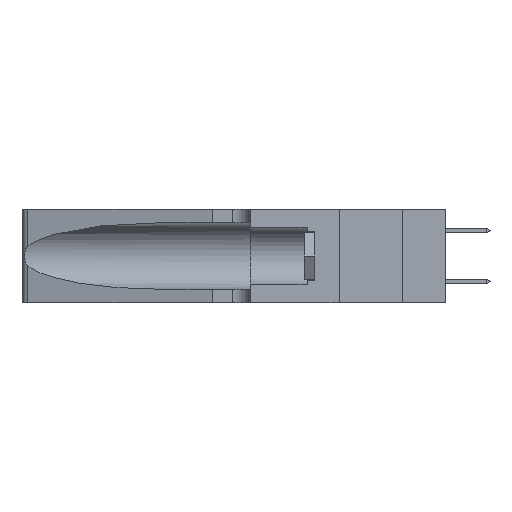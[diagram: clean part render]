
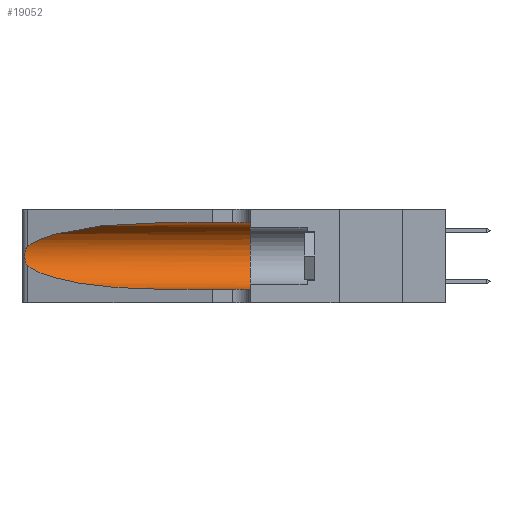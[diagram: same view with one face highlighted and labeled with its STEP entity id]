
A CAD part, left-side view. The second image highlights one B-rep face of the part: STEP entity #19052.
In plain terms, the highlighted cylindrical face has radius 3.308 mm (diameter 6.617 mm), a partial arc.
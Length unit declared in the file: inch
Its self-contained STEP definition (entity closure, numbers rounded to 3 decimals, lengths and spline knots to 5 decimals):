
#151 =( BOUNDED_CURVE ( )  B_SPLINE_CURVE ( 3, ( #10695, #19587, #8833, #23328 ),
 .UNSPECIFIED., .F., .T. ) 
 B_SPLINE_CURVE_WITH_KNOTS ( ( 4, 4 ),
 ( 1.5708, 2.84003 ),
 .UNSPECIFIED. ) 
 CURVE ( )  GEOMETRIC_REPRESENTATION_ITEM ( )  RATIONAL_B_SPLINE_CURVE ( ( 1., 0.87, 0.87, 1. ) ) 
 REPRESENTATION_ITEM ( '' )  );
#840 = CIRCLE ( 'NONE', #18734, 0.13025 ) ;
#911 =( BOUNDED_CURVE ( )  B_SPLINE_CURVE ( 3, ( #17438, #15646, #2801, #6527 ),
 .UNSPECIFIED., .F., .F. ) 
 B_SPLINE_CURVE_WITH_KNOTS ( ( 4, 4 ),
 ( 3.44316, 4.71239 ),
 .UNSPECIFIED. ) 
 CURVE ( )  GEOMETRIC_REPRESENTATION_ITEM ( )  RATIONAL_B_SPLINE_CURVE ( ( 1., 0.87, 0.87, 1. ) ) 
 REPRESENTATION_ITEM ( '' )  );
#1619 = LINE ( 'NONE', #19069, #5985 ) ;
#1751 = CARTESIAN_POINT ( 'NONE',  ( 0.1305, 0.35, 0.05475 ) ) ;
#1871 = CARTESIAN_POINT ( 'NONE',  ( 0.25639, 1.23186, 0.15144 ) ) ;
#2801 = CARTESIAN_POINT ( 'NONE',  ( 0.18966, 0.96281, 0.05475 ) ) ;
#3172 = VECTOR ( 'NONE', #9650, 39.37008 ) ;
#3465 = CYLINDRICAL_SURFACE ( 'NONE', #13192, 0.13025 ) ;
#3739 = CARTESIAN_POINT ( 'NONE',  ( 0.25487, 1.22718, 0.14631 ) ) ;
#3909 = CARTESIAN_POINT ( 'NONE',  ( 0.25856, 1.23593, 0.16098 ) ) ;
#3987 = ORIENTED_EDGE ( 'NONE', *, *, #12861, .F. ) ;
#4538 = CARTESIAN_POINT ( 'NONE',  ( 0.1305, 0.35, 0.185 ) ) ;
#5388 = ORIENTED_EDGE ( 'NONE', *, *, #22211, .T. ) ;
#5521 = CARTESIAN_POINT ( 'NONE',  ( 0.25639, 1.23184, 0.21858 ) ) ;
#5745 = EDGE_CURVE ( 'NONE', #7766, #9143, #911, .T. ) ;
#5985 = VECTOR ( 'NONE', #10089, 39.37008 ) ;
#6238 = CARTESIAN_POINT ( 'NONE',  ( 0.25487, 1.22718, 0.14631 ) ) ;
#6394 = DIRECTION ( 'NONE',  ( 0., 0., 1. ) ) ;
#6527 = CARTESIAN_POINT ( 'NONE',  ( 0.1305, 0.72297, 0.05475 ) ) ;
#6987 = DIRECTION ( 'NONE',  ( 0., -1., 0. ) ) ;
#7397 = CARTESIAN_POINT ( 'NONE',  ( 0.25854, 1.2359, 0.20912 ) ) ;
#7766 = VERTEX_POINT ( 'NONE', #6238 ) ;
#8833 = CARTESIAN_POINT ( 'NONE',  ( 0.2373, 1.15595, 0.28018 ) ) ;
#8874 = CARTESIAN_POINT ( 'NONE',  ( 0.25487, 1.22718, 0.22369 ) ) ;
#9143 = VERTEX_POINT ( 'NONE', #17431 ) ;
#9253 = CARTESIAN_POINT ( 'NONE',  ( 0.26075, 1.23896, 0.19203 ) ) ;
#9650 = DIRECTION ( 'NONE',  ( 0., -1., 0. ) ) ;
#10089 = DIRECTION ( 'NONE',  ( 0., -1., 0. ) ) ;
#10695 = CARTESIAN_POINT ( 'NONE',  ( 0.1305, 0.72297, 0.31525 ) ) ;
#10703 = CARTESIAN_POINT ( 'NONE',  ( 0.1305, 1.61858, 0.185 ) ) ;
#11000 = ORIENTED_EDGE ( 'NONE', *, *, #19455, .F. ) ;
#11032 = CARTESIAN_POINT ( 'NONE',  ( 0.25555, 1.22994, 0.2215 ) ) ;
#11114 = CARTESIAN_POINT ( 'NONE',  ( 0.26017, 1.23833, 0.17102 ) ) ;
#11412 = ORIENTED_EDGE ( 'NONE', *, *, #19323, .T. ) ;
#11807 = EDGE_CURVE ( 'NONE', #14571, #14377, #151, .T. ) ;
#12861 = EDGE_CURVE ( 'NONE', #14571, #17316, #1619, .T. ) ;
#12938 = CARTESIAN_POINT ( 'NONE',  ( 0.25789, 1.23486, 0.15765 ) ) ;
#13192 = AXIS2_PLACEMENT_3D ( 'NONE', #10703, #6987, #19671 ) ;
#13680 = ORIENTED_EDGE ( 'NONE', *, *, #11807, .T. ) ;
#14377 = VERTEX_POINT ( 'NONE', #8874 ) ;
#14571 = VERTEX_POINT ( 'NONE', #22002 ) ;
#14753 = CARTESIAN_POINT ( 'NONE',  ( 0.25555, 1.22993, 0.14849 ) ) ;
#15646 = CARTESIAN_POINT ( 'NONE',  ( 0.2373, 1.15595, 0.08982 ) ) ;
#15791 = EDGE_LOOP ( 'NONE', ( #13680, #5388, #15942, #11412, #11000, #3987 ) ) ;
#15942 = ORIENTED_EDGE ( 'NONE', *, *, #5745, .T. ) ;
#17316 = VERTEX_POINT ( 'NONE', #18749 ) ;
#17317 = DIRECTION ( 'NONE',  ( 0., 1., 0. ) ) ;
#17431 = CARTESIAN_POINT ( 'NONE',  ( 0.1305, 0.72297, 0.05475 ) ) ;
#17438 = CARTESIAN_POINT ( 'NONE',  ( 0.25487, 1.22718, 0.14631 ) ) ;
#18033 = FACE_OUTER_BOUND ( 'NONE', #15791, .T. ) ;
#18049 = B_SPLINE_CURVE_WITH_KNOTS ( 'NONE', 3,
 ( #23655, #11032, #5521, #18255, #7397, #20076, #9253, #21914, #11114, #3909, #12938, #1871, #14753, #3739 ),
 .UNSPECIFIED., .F., .F.,
 ( 4, 2, 2, 2, 2, 2, 4 ),
 ( 0., 0.00027, 0.00053, 0.00107, 0.0016, 0.00187, 0.00214 ),
 .UNSPECIFIED. ) ;
#18255 = CARTESIAN_POINT ( 'NONE',  ( 0.25787, 1.23484, 0.2124 ) ) ;
#18734 = AXIS2_PLACEMENT_3D ( 'NONE', #4538, #17317, #6394 ) ;
#18749 = CARTESIAN_POINT ( 'NONE',  ( 0.1305, 0.35, 0.31525 ) ) ;
#19052 = ADVANCED_FACE ( 'NONE', ( #18033 ), #3465, .F. ) ;
#19069 = CARTESIAN_POINT ( 'NONE',  ( 0.1305, 1.61858, 0.31525 ) ) ;
#19323 = EDGE_CURVE ( 'NONE', #9143, #22773, #22578, .T. ) ;
#19455 = EDGE_CURVE ( 'NONE', #17316, #22773, #840, .T. ) ;
#19587 = CARTESIAN_POINT ( 'NONE',  ( 0.18966, 0.96281, 0.31525 ) ) ;
#19671 = DIRECTION ( 'NONE',  ( 0., 0., -1. ) ) ;
#20076 = CARTESIAN_POINT ( 'NONE',  ( 0.26018, 1.23835, 0.19895 ) ) ;
#21914 = CARTESIAN_POINT ( 'NONE',  ( 0.26075, 1.23896, 0.178 ) ) ;
#22002 = CARTESIAN_POINT ( 'NONE',  ( 0.1305, 0.72297, 0.31525 ) ) ;
#22211 = EDGE_CURVE ( 'NONE', #14377, #7766, #18049, .T. ) ;
#22294 = CARTESIAN_POINT ( 'NONE',  ( 0.1305, 1.61858, 0.05475 ) ) ;
#22578 = LINE ( 'NONE', #22294, #3172 ) ;
#22773 = VERTEX_POINT ( 'NONE', #1751 ) ;
#23328 = CARTESIAN_POINT ( 'NONE',  ( 0.25487, 1.22718, 0.22369 ) ) ;
#23655 = CARTESIAN_POINT ( 'NONE',  ( 0.25487, 1.22718, 0.22369 ) ) ;
